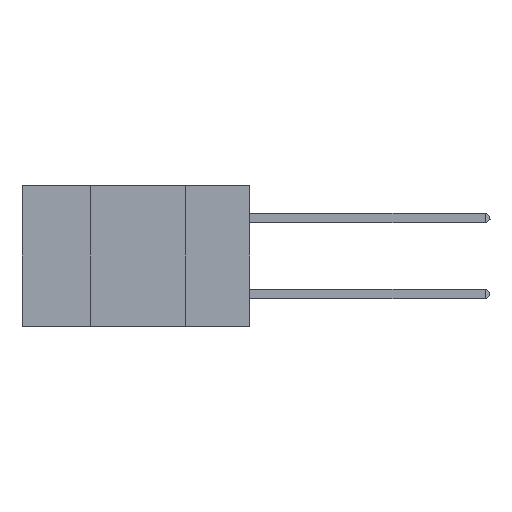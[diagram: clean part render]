
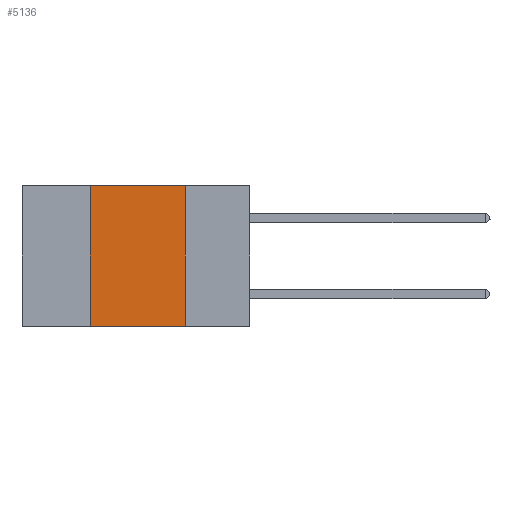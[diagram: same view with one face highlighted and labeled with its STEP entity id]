
A CAD part, left-side view. The second image highlights one B-rep face of the part: STEP entity #5136.
In plain terms, the highlighted planar face has unit normal (-1, 0, 0).
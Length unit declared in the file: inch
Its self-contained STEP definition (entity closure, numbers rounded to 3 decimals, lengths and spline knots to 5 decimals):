
#19 = PLANE ( 'NONE',  #3252 ) ;
#148 = DIRECTION ( 'NONE',  ( 0., 0., -1. ) ) ;
#396 = ORIENTED_EDGE ( 'NONE', *, *, #17096, .T. ) ;
#1311 = DIRECTION ( 'NONE',  ( 0., 0., 1. ) ) ;
#1561 = VECTOR ( 'NONE', #1311, 39.37008 ) ;
#1659 = CARTESIAN_POINT ( 'NONE',  ( 0., 0.17, 0. ) ) ;
#3252 = AXIS2_PLACEMENT_3D ( 'NONE', #12968, #16646, #148 ) ;
#3477 = CARTESIAN_POINT ( 'NONE',  ( 0., 0.42, 0. ) ) ;
#4023 = DIRECTION ( 'NONE',  ( 0., -1., 0. ) ) ;
#4087 = EDGE_CURVE ( 'NONE', #19292, #23599, #23520, .T. ) ;
#4259 = CARTESIAN_POINT ( 'NONE',  ( 0., 0.6, -0.37 ) ) ;
#4979 = CARTESIAN_POINT ( 'NONE',  ( 0., 0.17, -0.37 ) ) ;
#5069 = VECTOR ( 'NONE', #14519, 39.37008 ) ;
#5136 = ADVANCED_FACE ( 'NONE', ( #16530 ), #19, .F. ) ;
#5412 = DIRECTION ( 'NONE',  ( 0., -1., 0. ) ) ;
#5591 = ORIENTED_EDGE ( 'NONE', *, *, #4087, .F. ) ;
#6162 = EDGE_CURVE ( 'NONE', #14404, #19292, #11106, .T. ) ;
#7001 = CARTESIAN_POINT ( 'NONE',  ( 0., 0.42, 0. ) ) ;
#7971 = ORIENTED_EDGE ( 'NONE', *, *, #20684, .F. ) ;
#11106 = LINE ( 'NONE', #16705, #14001 ) ;
#11454 = VECTOR ( 'NONE', #4023, 39.37008 ) ;
#12430 = LINE ( 'NONE', #7001, #1561 ) ;
#12968 = CARTESIAN_POINT ( 'NONE',  ( 0., 0.6, 0. ) ) ;
#14001 = VECTOR ( 'NONE', #5412, 39.37008 ) ;
#14404 = VERTEX_POINT ( 'NONE', #3477 ) ;
#14519 = DIRECTION ( 'NONE',  ( 0., 0., -1. ) ) ;
#15744 = ORIENTED_EDGE ( 'NONE', *, *, #6162, .F. ) ;
#16530 = FACE_OUTER_BOUND ( 'NONE', #17400, .T. ) ;
#16646 = DIRECTION ( 'NONE',  ( 1., 0., 0. ) ) ;
#16705 = CARTESIAN_POINT ( 'NONE',  ( 0., 0.6, 0. ) ) ;
#17096 = EDGE_CURVE ( 'NONE', #23083, #23599, #20514, .T. ) ;
#17400 = EDGE_LOOP ( 'NONE', ( #5591, #15744, #7971, #396 ) ) ;
#19292 = VERTEX_POINT ( 'NONE', #1659 ) ;
#19797 = CARTESIAN_POINT ( 'NONE',  ( 0., 0.42, -0.37 ) ) ;
#20514 = LINE ( 'NONE', #4259, #11454 ) ;
#20684 = EDGE_CURVE ( 'NONE', #23083, #14404, #12430, .T. ) ;
#21844 = CARTESIAN_POINT ( 'NONE',  ( 0., 0.17, 0. ) ) ;
#23083 = VERTEX_POINT ( 'NONE', #19797 ) ;
#23520 = LINE ( 'NONE', #21844, #5069 ) ;
#23599 = VERTEX_POINT ( 'NONE', #4979 ) ;
